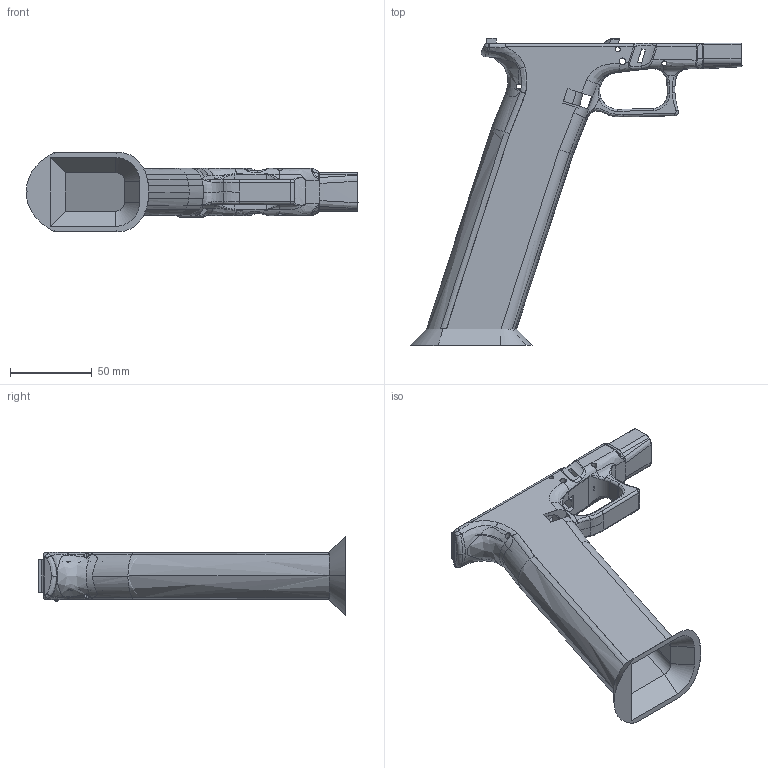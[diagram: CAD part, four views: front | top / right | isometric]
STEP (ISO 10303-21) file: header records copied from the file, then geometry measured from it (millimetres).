
FILE_DESCRIPTION (( 'STEP AP214' ), '1' );
FILE_NAME ('BidenHander_NoText.STEP', '2021-04-30T22:00:33', ( '' ), ( '' ), 'SwSTEP 2.0', 'SolidWorks 2019', '' );
FILE_SCHEMA (( 'AUTOMOTIVE_DESIGN' ));
Length unit declared in the file: millimetre
Products named in the file (1): BidenHander_NoText
Bounding box: 202.87 x 187.55 x 48.8 mm (x, y, z)
Volume: 134365.9 mm3; surface area: 68394.3 mm2
Topology: 1 solids, 3 shells, 598 faces, 1783 edges, 1139 vertices
Faces by surface type: bspline 259, plane 159, cylinder 155, torus 15, cone 10
Entity records: 42268 total; most frequent: CARTESIAN_POINT 29020, ORIENTED_EDGE 3502, EDGE_CURVE 1751, DIRECTION 1728, VERTEX_POINT 1139, B_SPLINE_CURVE_WITH_KNOTS 840, EDGE_LOOP 608, FACE_OUTER_BOUND 598
